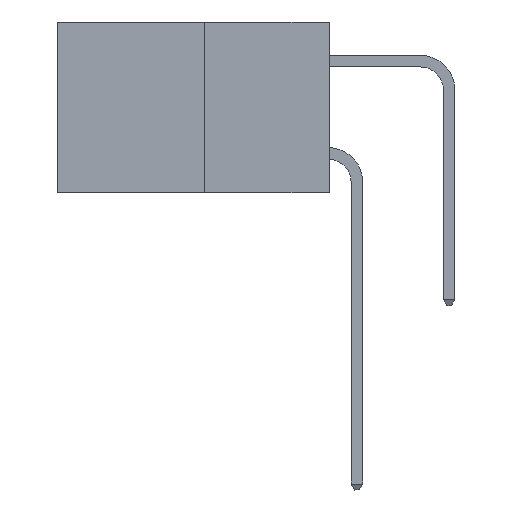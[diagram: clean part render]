
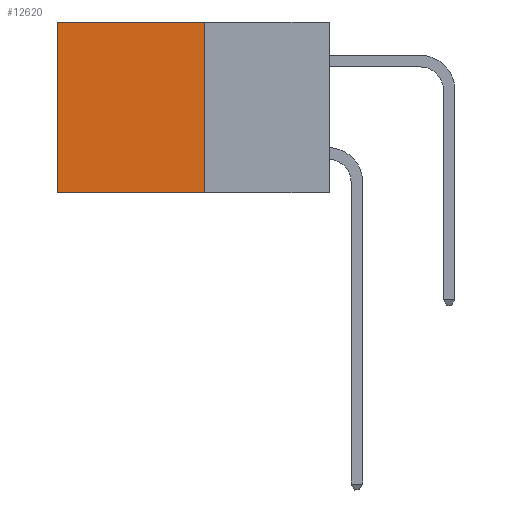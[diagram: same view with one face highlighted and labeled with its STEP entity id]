
A CAD part, left-side view. The second image highlights one B-rep face of the part: STEP entity #12620.
In plain terms, the highlighted planar face has unit normal (-1, 0, 0).
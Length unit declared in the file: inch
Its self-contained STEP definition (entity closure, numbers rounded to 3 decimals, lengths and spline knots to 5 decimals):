
#392 = EDGE_CURVE ( 'NONE', #1749, #1494, #13347, .T. ) ;
#607 = FACE_OUTER_BOUND ( 'NONE', #6713, .T. ) ;
#694 = CARTESIAN_POINT ( 'NONE',  ( 0.277, 0.59, -0.37 ) ) ;
#931 = VERTEX_POINT ( 'NONE', #4114 ) ;
#1494 = VERTEX_POINT ( 'NONE', #10973 ) ;
#1743 = VECTOR ( 'NONE', #13428, 39.37008 ) ;
#1749 = VERTEX_POINT ( 'NONE', #13020 ) ;
#1846 = DIRECTION ( 'NONE',  ( 0., 0., -1. ) ) ;
#1863 = CARTESIAN_POINT ( 'NONE',  ( 0.277, 0.27, -0.37 ) ) ;
#3213 = ORIENTED_EDGE ( 'NONE', *, *, #9294, .F. ) ;
#3318 = VECTOR ( 'NONE', #12146, 39.37008 ) ;
#3682 = LINE ( 'NONE', #5393, #3318 ) ;
#4114 = CARTESIAN_POINT ( 'NONE',  ( 0.277, 0.59, 0. ) ) ;
#4290 = VERTEX_POINT ( 'NONE', #10078 ) ;
#4813 = AXIS2_PLACEMENT_3D ( 'NONE', #11308, #12414, #5670 ) ;
#5393 = CARTESIAN_POINT ( 'NONE',  ( 0.277, 0.27, 0. ) ) ;
#5670 = DIRECTION ( 'NONE',  ( 0., 0., -1. ) ) ;
#6713 = EDGE_LOOP ( 'NONE', ( #12028, #3213, #7650, #10011 ) ) ;
#7034 = DIRECTION ( 'NONE',  ( 0., 1., 0. ) ) ;
#7374 = VECTOR ( 'NONE', #1846, 39.37008 ) ;
#7650 = ORIENTED_EDGE ( 'NONE', *, *, #392, .F. ) ;
#7753 = LINE ( 'NONE', #694, #7374 ) ;
#7911 = PLANE ( 'NONE',  #4813 ) ;
#9294 = EDGE_CURVE ( 'NONE', #1494, #4290, #13724, .T. ) ;
#10011 = ORIENTED_EDGE ( 'NONE', *, *, #13854, .T. ) ;
#10078 = CARTESIAN_POINT ( 'NONE',  ( 0.277, 0.59, -0.37 ) ) ;
#10894 = VECTOR ( 'NONE', #7034, 39.37008 ) ;
#10973 = CARTESIAN_POINT ( 'NONE',  ( 0.277, 0.27, -0.37 ) ) ;
#11308 = CARTESIAN_POINT ( 'NONE',  ( 0.277, 0.27, -0.37 ) ) ;
#11526 = CARTESIAN_POINT ( 'NONE',  ( 0.277, 0.27, -0.37 ) ) ;
#12028 = ORIENTED_EDGE ( 'NONE', *, *, #13772, .T. ) ;
#12146 = DIRECTION ( 'NONE',  ( 0., 1., 0. ) ) ;
#12414 = DIRECTION ( 'NONE',  ( 1., 0., 0. ) ) ;
#12620 = ADVANCED_FACE ( 'NONE', ( #607 ), #7911, .F. ) ;
#13020 = CARTESIAN_POINT ( 'NONE',  ( 0.277, 0.27, 0. ) ) ;
#13347 = LINE ( 'NONE', #1863, #1743 ) ;
#13428 = DIRECTION ( 'NONE',  ( 0., 0., -1. ) ) ;
#13724 = LINE ( 'NONE', #11526, #10894 ) ;
#13772 = EDGE_CURVE ( 'NONE', #931, #4290, #7753, .T. ) ;
#13854 = EDGE_CURVE ( 'NONE', #1749, #931, #3682, .T. ) ;
